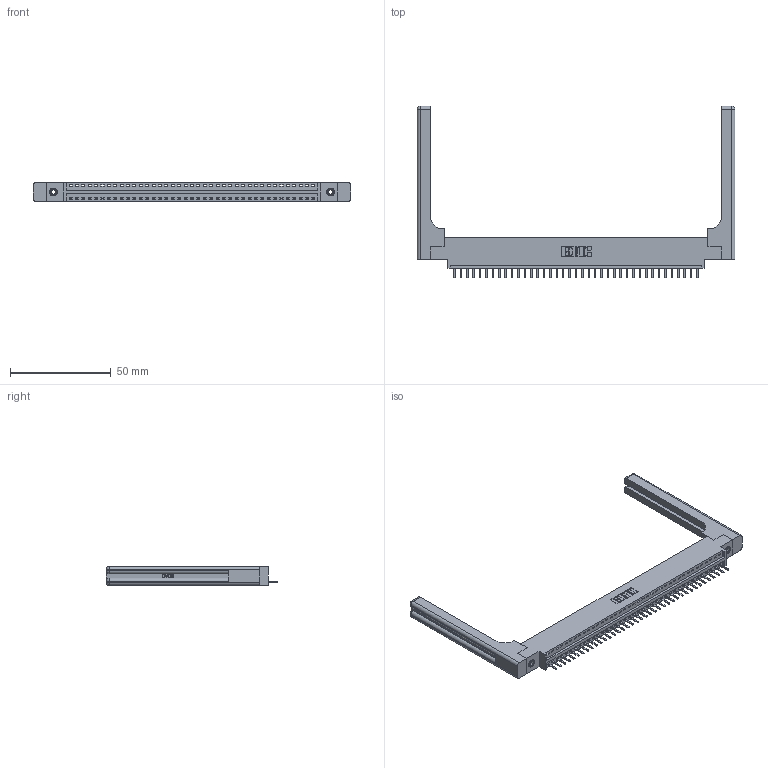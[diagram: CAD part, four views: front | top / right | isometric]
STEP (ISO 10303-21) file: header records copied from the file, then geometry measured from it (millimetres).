
FILE_DESCRIPTION (( 'STEP AP203' ), '1' );
FILE_NAME ('396-039-520-658.STEP', '2019-10-27T18:57:27', ( '' ), ( '' ), 'SwSTEP 2.0', 'SolidWorks 2016', '' );
FILE_SCHEMA (( 'CONFIG_CONTROL_DESIGN' ));
Length unit declared in the file: inch
Products named in the file (5): 346 Part_0.170 Offset - 0.156 Dia-TH; 396-039-520-658; 345-250-001_345-250-001-102; 346-220-058_345-220-058; 345-292-001_345-293-120
Assembly tree (44 placements, depth 2):
  396-039-520-658
    346 Part_0.170 Offset - 0.156 Dia-TH
    345-292-001_345-293-120  x39
    345-250-001_345-250-001-102  x2
    346-220-058_345-220-058  x2
Bounding box: 157.89 x 85.29 x 9.4 mm (x, y, z)
Volume: 22344.1 mm3; surface area: 23453.3 mm2
Topology: 44 solids, 44 shells, 2800 faces, 8183 edges, 5330 vertices
Faces by surface type: plane 1866, cylinder 874, bspline 36, cone 12, sphere 8, torus 4
Entity records: 30036 total; most frequent: CARTESIAN_POINT 6142, ORIENTED_EDGE 4900, DIRECTION 4340, EDGE_CURVE 2450, LINE 2066, VECTOR 2066, VERTEX_POINT 1622, AXIS2_PLACEMENT_3D 1137
